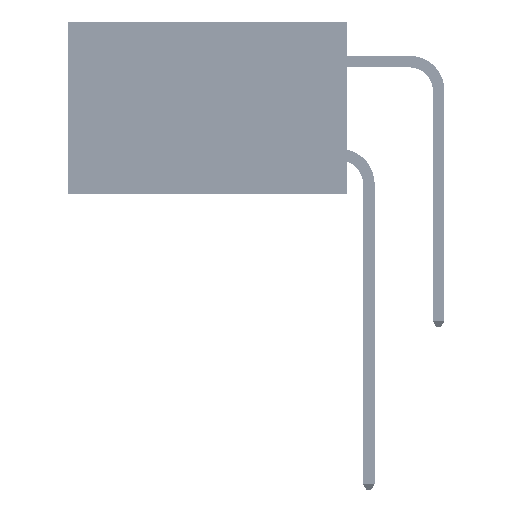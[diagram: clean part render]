
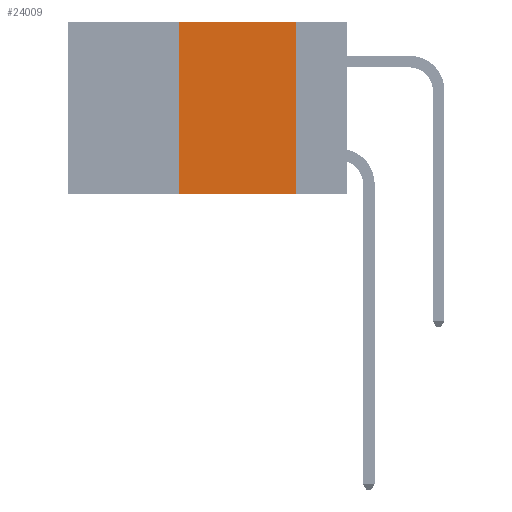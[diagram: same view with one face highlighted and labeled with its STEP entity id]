
A CAD part, left-side view. The second image highlights one B-rep face of the part: STEP entity #24009.
In plain terms, the highlighted planar face has unit normal (-1, 0, 0).
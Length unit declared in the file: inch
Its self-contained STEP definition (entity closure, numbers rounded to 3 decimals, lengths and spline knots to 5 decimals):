
#3459 = PLANE ( 'NONE',  #43077 ) ;
#4499 = VECTOR ( 'NONE', #31594, 39.37008 ) ;
#4655 = EDGE_LOOP ( 'NONE', ( #39169, #48926, #5749, #47216 ) ) ;
#5749 = ORIENTED_EDGE ( 'NONE', *, *, #27598, .F. ) ;
#5952 = CARTESIAN_POINT ( 'NONE',  ( 0., 0.6, -0.37 ) ) ;
#7363 = CARTESIAN_POINT ( 'NONE',  ( 0., 0.6, 0. ) ) ;
#7583 = VERTEX_POINT ( 'NONE', #50145 ) ;
#10475 = LINE ( 'NONE', #39353, #49911 ) ;
#11598 = DIRECTION ( 'NONE',  ( 0., 0., -1. ) ) ;
#11640 = FACE_OUTER_BOUND ( 'NONE', #4655, .T. ) ;
#13047 = VECTOR ( 'NONE', #29680, 39.37008 ) ;
#15642 = EDGE_CURVE ( 'NONE', #41181, #41451, #27208, .T. ) ;
#16593 = CARTESIAN_POINT ( 'NONE',  ( 0., 0.36, -0.37 ) ) ;
#19280 = CARTESIAN_POINT ( 'NONE',  ( 0., 0.6, 0. ) ) ;
#24009 = ADVANCED_FACE ( 'NONE', ( #11640 ), #3459, .F. ) ;
#25406 = LINE ( 'NONE', #50919, #4499 ) ;
#26238 = VECTOR ( 'NONE', #31276, 39.37008 ) ;
#27208 = LINE ( 'NONE', #5952, #13047 ) ;
#27598 = EDGE_CURVE ( 'NONE', #41181, #46419, #25406, .T. ) ;
#29680 = DIRECTION ( 'NONE',  ( 0., -1., 0. ) ) ;
#30958 = DIRECTION ( 'NONE',  ( 1., 0., 0. ) ) ;
#31125 = DIRECTION ( 'NONE',  ( 0., 0., -1. ) ) ;
#31276 = DIRECTION ( 'NONE',  ( 0., -1., 0. ) ) ;
#31594 = DIRECTION ( 'NONE',  ( 0., 0., 1. ) ) ;
#36316 = EDGE_CURVE ( 'NONE', #7583, #41451, #10475, .T. ) ;
#36772 = LINE ( 'NONE', #7363, #26238 ) ;
#38832 = EDGE_CURVE ( 'NONE', #46419, #7583, #36772, .T. ) ;
#39169 = ORIENTED_EDGE ( 'NONE', *, *, #36316, .F. ) ;
#39353 = CARTESIAN_POINT ( 'NONE',  ( 0., 0.11, 0. ) ) ;
#41181 = VERTEX_POINT ( 'NONE', #16593 ) ;
#41451 = VERTEX_POINT ( 'NONE', #46403 ) ;
#43077 = AXIS2_PLACEMENT_3D ( 'NONE', #19280, #30958, #31125 ) ;
#43850 = CARTESIAN_POINT ( 'NONE',  ( 0., 0.36, 0. ) ) ;
#46403 = CARTESIAN_POINT ( 'NONE',  ( 0., 0.11, -0.37 ) ) ;
#46419 = VERTEX_POINT ( 'NONE', #43850 ) ;
#47216 = ORIENTED_EDGE ( 'NONE', *, *, #15642, .T. ) ;
#48926 = ORIENTED_EDGE ( 'NONE', *, *, #38832, .F. ) ;
#49911 = VECTOR ( 'NONE', #11598, 39.37008 ) ;
#50145 = CARTESIAN_POINT ( 'NONE',  ( 0., 0.11, 0. ) ) ;
#50919 = CARTESIAN_POINT ( 'NONE',  ( 0., 0.36, 0. ) ) ;
